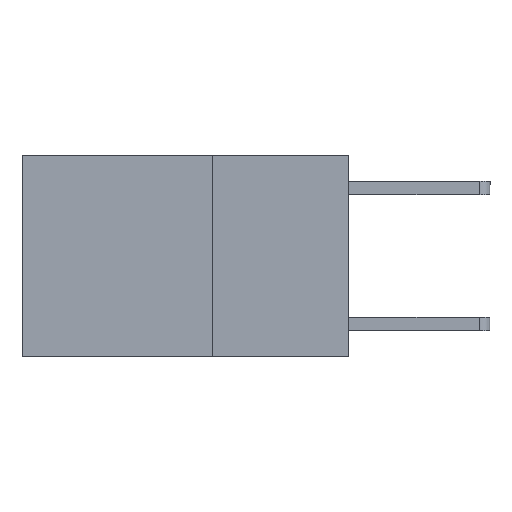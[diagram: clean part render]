
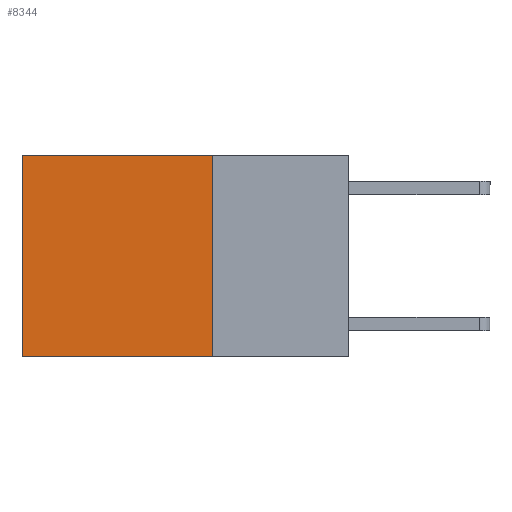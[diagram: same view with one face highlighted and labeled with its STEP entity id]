
A CAD part, left-side view. The second image highlights one B-rep face of the part: STEP entity #8344.
In plain terms, the highlighted planar face has unit normal (-1, 0, 0).
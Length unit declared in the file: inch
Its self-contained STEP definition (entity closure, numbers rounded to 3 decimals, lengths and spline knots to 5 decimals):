
#35 = VERTEX_POINT ( 'NONE', #795 ) ;
#758 = ORIENTED_EDGE ( 'NONE', *, *, #7519, .F. ) ;
#795 = CARTESIAN_POINT ( 'NONE',  ( 0.2625, 0.25, 0. ) ) ;
#836 = VECTOR ( 'NONE', #3063, 39.37008 ) ;
#1380 = ORIENTED_EDGE ( 'NONE', *, *, #2940, .F. ) ;
#2240 = PLANE ( 'NONE',  #4807 ) ;
#2374 = VECTOR ( 'NONE', #9117, 39.37008 ) ;
#2485 = LINE ( 'NONE', #3261, #8709 ) ;
#2596 = DIRECTION ( 'NONE',  ( 0., 1., 0. ) ) ;
#2923 = EDGE_LOOP ( 'NONE', ( #8666, #758, #1380, #5786 ) ) ;
#2940 = EDGE_CURVE ( 'NONE', #35, #6106, #2959, .T. ) ;
#2959 = LINE ( 'NONE', #6766, #836 ) ;
#3063 = DIRECTION ( 'NONE',  ( 0., 0., -1. ) ) ;
#3103 = EDGE_CURVE ( 'NONE', #35, #7400, #2485, .T. ) ;
#3261 = CARTESIAN_POINT ( 'NONE',  ( 0.2625, 0.25, 0. ) ) ;
#4049 = EDGE_CURVE ( 'NONE', #7400, #5065, #7600, .T. ) ;
#4276 = DIRECTION ( 'NONE',  ( 0., 1., 0. ) ) ;
#4362 = CARTESIAN_POINT ( 'NONE',  ( 0.2625, 0.25, -0.37 ) ) ;
#4807 = AXIS2_PLACEMENT_3D ( 'NONE', #6665, #7405, #5079 ) ;
#5065 = VERTEX_POINT ( 'NONE', #8673 ) ;
#5079 = DIRECTION ( 'NONE',  ( 0., 0., -1. ) ) ;
#5466 = CARTESIAN_POINT ( 'NONE',  ( 0.2625, 0.6, 0. ) ) ;
#5786 = ORIENTED_EDGE ( 'NONE', *, *, #3103, .T. ) ;
#6106 = VERTEX_POINT ( 'NONE', #8366 ) ;
#6176 = VECTOR ( 'NONE', #4276, 39.37008 ) ;
#6606 = FACE_OUTER_BOUND ( 'NONE', #2923, .T. ) ;
#6665 = CARTESIAN_POINT ( 'NONE',  ( 0.2625, 0.25, 0. ) ) ;
#6766 = CARTESIAN_POINT ( 'NONE',  ( 0.2625, 0.25, 0. ) ) ;
#7170 = LINE ( 'NONE', #4362, #6176 ) ;
#7400 = VERTEX_POINT ( 'NONE', #7827 ) ;
#7405 = DIRECTION ( 'NONE',  ( 1., 0., 0. ) ) ;
#7519 = EDGE_CURVE ( 'NONE', #6106, #5065, #7170, .T. ) ;
#7600 = LINE ( 'NONE', #5466, #2374 ) ;
#7827 = CARTESIAN_POINT ( 'NONE',  ( 0.2625, 0.6, 0. ) ) ;
#8344 = ADVANCED_FACE ( 'NONE', ( #6606 ), #2240, .F. ) ;
#8366 = CARTESIAN_POINT ( 'NONE',  ( 0.2625, 0.25, -0.37 ) ) ;
#8666 = ORIENTED_EDGE ( 'NONE', *, *, #4049, .T. ) ;
#8673 = CARTESIAN_POINT ( 'NONE',  ( 0.2625, 0.6, -0.37 ) ) ;
#8709 = VECTOR ( 'NONE', #2596, 39.37008 ) ;
#9117 = DIRECTION ( 'NONE',  ( 0., 0., -1. ) ) ;
